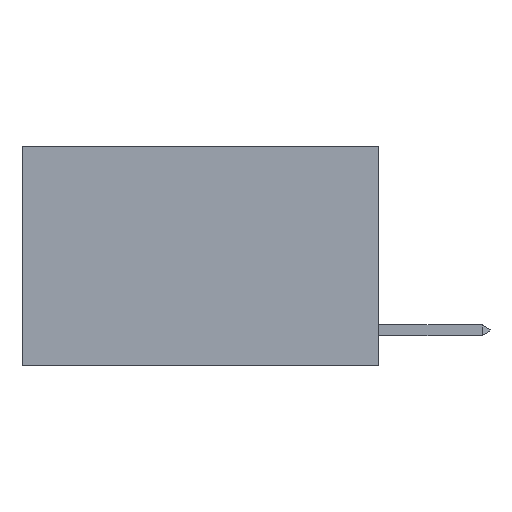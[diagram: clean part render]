
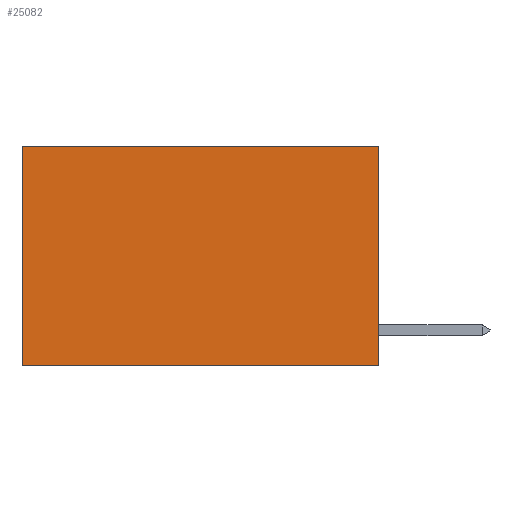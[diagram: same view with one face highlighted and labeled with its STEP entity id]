
A CAD part, left-side view. The second image highlights one B-rep face of the part: STEP entity #25082.
In plain terms, the highlighted planar face has unit normal (-1, 0, 0).
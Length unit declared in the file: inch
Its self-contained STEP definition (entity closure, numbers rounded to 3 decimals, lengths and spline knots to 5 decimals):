
#727 = DIRECTION ( 'NONE',  ( 0., 1., 0. ) ) ;
#985 = DIRECTION ( 'NONE',  ( 1., 0., 0. ) ) ;
#1757 = CARTESIAN_POINT ( 'NONE',  ( 0.2625, 0.6, 0. ) ) ;
#1811 = CARTESIAN_POINT ( 'NONE',  ( 0.2625, 0., 0. ) ) ;
#2329 = VERTEX_POINT ( 'NONE', #11871 ) ;
#4469 = CARTESIAN_POINT ( 'NONE',  ( 0.2625, 0., -0.37 ) ) ;
#4478 = AXIS2_PLACEMENT_3D ( 'NONE', #21242, #985, #11248 ) ;
#4671 = LINE ( 'NONE', #12790, #19471 ) ;
#5015 = PLANE ( 'NONE',  #4478 ) ;
#5955 = DIRECTION ( 'NONE',  ( 0., 1., 0. ) ) ;
#6011 = VECTOR ( 'NONE', #5955, 39.37008 ) ;
#6931 = LINE ( 'NONE', #15246, #17812 ) ;
#8328 = EDGE_CURVE ( 'NONE', #26666, #10478, #18196, .T. ) ;
#9280 = ORIENTED_EDGE ( 'NONE', *, *, #8328, .F. ) ;
#9981 = EDGE_LOOP ( 'NONE', ( #24752, #22672, #9280, #10201 ) ) ;
#10201 = ORIENTED_EDGE ( 'NONE', *, *, #12517, .T. ) ;
#10478 = VERTEX_POINT ( 'NONE', #4469 ) ;
#11248 = DIRECTION ( 'NONE',  ( 0., 0., -1. ) ) ;
#11633 = CARTESIAN_POINT ( 'NONE',  ( 0.2625, 0., 0. ) ) ;
#11768 = DIRECTION ( 'NONE',  ( 0., 0., -1. ) ) ;
#11871 = CARTESIAN_POINT ( 'NONE',  ( 0.2625, 0.6, -0.37 ) ) ;
#12517 = EDGE_CURVE ( 'NONE', #26666, #23567, #24678, .T. ) ;
#12790 = CARTESIAN_POINT ( 'NONE',  ( 0.2625, 0.6, 0. ) ) ;
#15208 = EDGE_CURVE ( 'NONE', #10478, #2329, #6931, .T. ) ;
#15246 = CARTESIAN_POINT ( 'NONE',  ( 0.2625, 0., -0.37 ) ) ;
#15356 = FACE_OUTER_BOUND ( 'NONE', #9981, .T. ) ;
#17812 = VECTOR ( 'NONE', #727, 39.37008 ) ;
#18196 = LINE ( 'NONE', #11633, #24625 ) ;
#19378 = CARTESIAN_POINT ( 'NONE',  ( 0.2625, 0., 0. ) ) ;
#19471 = VECTOR ( 'NONE', #21158, 39.37008 ) ;
#21158 = DIRECTION ( 'NONE',  ( 0., 0., -1. ) ) ;
#21242 = CARTESIAN_POINT ( 'NONE',  ( 0.2625, 0., 0. ) ) ;
#22672 = ORIENTED_EDGE ( 'NONE', *, *, #15208, .F. ) ;
#23567 = VERTEX_POINT ( 'NONE', #1757 ) ;
#24625 = VECTOR ( 'NONE', #11768, 39.37008 ) ;
#24678 = LINE ( 'NONE', #1811, #6011 ) ;
#24752 = ORIENTED_EDGE ( 'NONE', *, *, #26609, .T. ) ;
#25082 = ADVANCED_FACE ( 'NONE', ( #15356 ), #5015, .F. ) ;
#26609 = EDGE_CURVE ( 'NONE', #23567, #2329, #4671, .T. ) ;
#26666 = VERTEX_POINT ( 'NONE', #19378 ) ;
